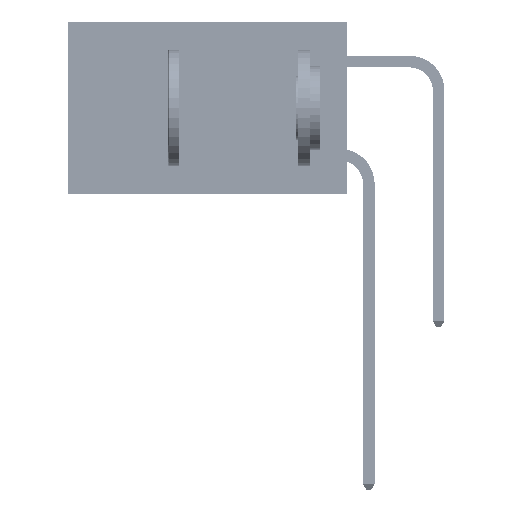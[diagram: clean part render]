
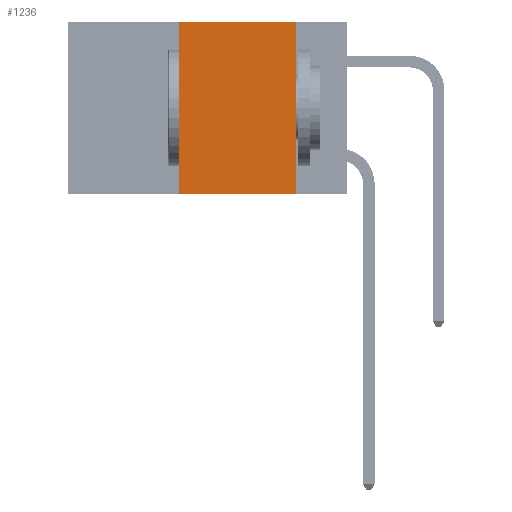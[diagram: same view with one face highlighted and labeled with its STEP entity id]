
A CAD part, left-side view. The second image highlights one B-rep face of the part: STEP entity #1236.
In plain terms, the highlighted planar face has unit normal (-1, 0, 0).
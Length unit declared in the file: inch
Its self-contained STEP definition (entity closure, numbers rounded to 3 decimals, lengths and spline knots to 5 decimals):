
#179 = VECTOR ( 'NONE', #7559, 39.37008 ) ;
#1158 = VECTOR ( 'NONE', #38991, 39.37008 ) ;
#1236 = ADVANCED_FACE ( 'NONE', ( #29798 ), #13506, .F. ) ;
#2049 = CARTESIAN_POINT ( 'NONE',  ( 0., 0.6, 0. ) ) ;
#4012 = VECTOR ( 'NONE', #21129, 39.37008 ) ;
#5029 = VERTEX_POINT ( 'NONE', #27656 ) ;
#5558 = EDGE_CURVE ( 'NONE', #24145, #5029, #31468, .T. ) ;
#7559 = DIRECTION ( 'NONE',  ( 0., -1., 0. ) ) ;
#9233 = DIRECTION ( 'NONE',  ( 1., 0., 0. ) ) ;
#12823 = AXIS2_PLACEMENT_3D ( 'NONE', #2049, #9233, #47097 ) ;
#13506 = PLANE ( 'NONE',  #12823 ) ;
#13964 = CARTESIAN_POINT ( 'NONE',  ( 0., 0.6, 0. ) ) ;
#14089 = LINE ( 'NONE', #13964, #4012 ) ;
#17117 = EDGE_CURVE ( 'NONE', #5029, #19702, #14089, .T. ) ;
#17981 = ORIENTED_EDGE ( 'NONE', *, *, #27563, .T. ) ;
#19499 = CARTESIAN_POINT ( 'NONE',  ( 0., 0.36, 0. ) ) ;
#19702 = VERTEX_POINT ( 'NONE', #41569 ) ;
#20062 = LINE ( 'NONE', #29681, #40173 ) ;
#21129 = DIRECTION ( 'NONE',  ( 0., -1., 0. ) ) ;
#23729 = VERTEX_POINT ( 'NONE', #37186 ) ;
#24145 = VERTEX_POINT ( 'NONE', #31555 ) ;
#27563 = EDGE_CURVE ( 'NONE', #24145, #23729, #37535, .T. ) ;
#27656 = CARTESIAN_POINT ( 'NONE',  ( 0., 0.36, 0. ) ) ;
#29681 = CARTESIAN_POINT ( 'NONE',  ( 0., 0.11, 0. ) ) ;
#29798 = FACE_OUTER_BOUND ( 'NONE', #35433, .T. ) ;
#31468 = LINE ( 'NONE', #19499, #1158 ) ;
#31555 = CARTESIAN_POINT ( 'NONE',  ( 0., 0.36, -0.37 ) ) ;
#34311 = ORIENTED_EDGE ( 'NONE', *, *, #47838, .F. ) ;
#34429 = CARTESIAN_POINT ( 'NONE',  ( 0., 0.6, -0.37 ) ) ;
#35433 = EDGE_LOOP ( 'NONE', ( #34311, #40900, #41577, #17981 ) ) ;
#37186 = CARTESIAN_POINT ( 'NONE',  ( 0., 0.11, -0.37 ) ) ;
#37535 = LINE ( 'NONE', #34429, #179 ) ;
#38991 = DIRECTION ( 'NONE',  ( 0., 0., 1. ) ) ;
#40173 = VECTOR ( 'NONE', #44506, 39.37008 ) ;
#40900 = ORIENTED_EDGE ( 'NONE', *, *, #17117, .F. ) ;
#41569 = CARTESIAN_POINT ( 'NONE',  ( 0., 0.11, 0. ) ) ;
#41577 = ORIENTED_EDGE ( 'NONE', *, *, #5558, .F. ) ;
#44506 = DIRECTION ( 'NONE',  ( 0., 0., -1. ) ) ;
#47097 = DIRECTION ( 'NONE',  ( 0., 0., -1. ) ) ;
#47838 = EDGE_CURVE ( 'NONE', #19702, #23729, #20062, .T. ) ;
